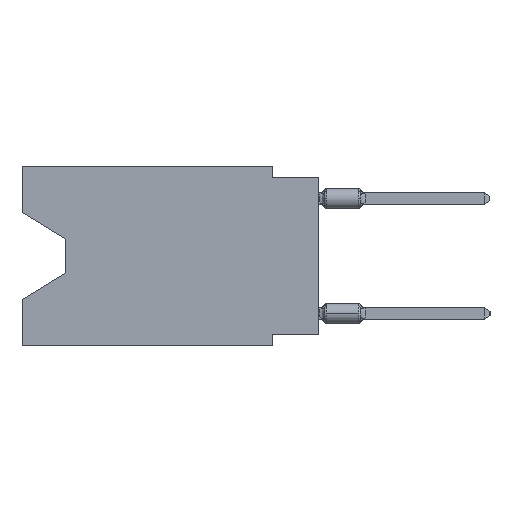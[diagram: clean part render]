
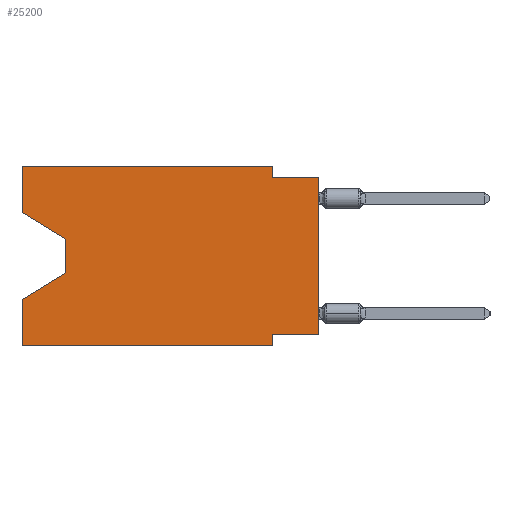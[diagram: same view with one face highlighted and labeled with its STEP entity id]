
A CAD part, left-side view. The second image highlights one B-rep face of the part: STEP entity #25200.
In plain terms, the highlighted planar face has unit normal (-1, 0, 0).
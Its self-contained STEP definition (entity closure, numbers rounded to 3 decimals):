
#260 = VECTOR ( 'NONE', #6667, 1000. ) ;
#454 = EDGE_CURVE ( 'NONE', #11448, #11130, #2234, .T. ) ;
#1502 = EDGE_CURVE ( 'NONE', #12271, #10239, #15780, .T. ) ;
#1909 = VECTOR ( 'NONE', #20679, 1000. ) ;
#2165 = ORIENTED_EDGE ( 'NONE', *, *, #1502, .T. ) ;
#2206 = ORIENTED_EDGE ( 'NONE', *, *, #2248, .F. ) ;
#2234 = LINE ( 'NONE', #36126, #32923 ) ;
#2248 = EDGE_CURVE ( 'NONE', #7473, #11448, #11424, .T. ) ;
#3458 = LINE ( 'NONE', #6251, #7971 ) ;
#4123 = ORIENTED_EDGE ( 'NONE', *, *, #14112, .F. ) ;
#4466 = CARTESIAN_POINT ( 'NONE',  ( 0., 13.97, -4.013 ) ) ;
#4873 = DIRECTION ( 'NONE',  ( 0., 0., -1. ) ) ;
#5042 = VECTOR ( 'NONE', #34159, 1000. ) ;
#5079 = VECTOR ( 'NONE', #7875, 1000. ) ;
#5109 = CARTESIAN_POINT ( 'NONE',  ( 0., 16.383, -2.546 ) ) ;
#5145 = EDGE_CURVE ( 'NONE', #11130, #29030, #25120, .T. ) ;
#5317 = CARTESIAN_POINT ( 'NONE',  ( 0., 13.97, -5.893 ) ) ;
#6251 = CARTESIAN_POINT ( 'NONE',  ( 0., 16.383, 0. ) ) ;
#6667 = DIRECTION ( 'NONE',  ( 0., -1., 0. ) ) ;
#6865 = LINE ( 'NONE', #12619, #1909 ) ;
#7071 = DIRECTION ( 'NONE',  ( 0., 0., -1. ) ) ;
#7473 = VERTEX_POINT ( 'NONE', #35876 ) ;
#7667 = CARTESIAN_POINT ( 'NONE',  ( 0., 16.383, -7.36 ) ) ;
#7672 = DIRECTION ( 'NONE',  ( 1., 0., 0. ) ) ;
#7689 = VERTEX_POINT ( 'NONE', #17421 ) ;
#7839 = DIRECTION ( 'NONE',  ( 0., 0., -1. ) ) ;
#7875 = DIRECTION ( 'NONE',  ( 0., 1., 0. ) ) ;
#7919 = CARTESIAN_POINT ( 'NONE',  ( 0., 2.54, -9.906 ) ) ;
#7971 = VECTOR ( 'NONE', #25437, 1000. ) ;
#8649 = LINE ( 'NONE', #5317, #36386 ) ;
#10239 = VERTEX_POINT ( 'NONE', #7919 ) ;
#10853 = LINE ( 'NONE', #14024, #5079 ) ;
#11130 = VERTEX_POINT ( 'NONE', #29367 ) ;
#11178 = ORIENTED_EDGE ( 'NONE', *, *, #29796, .T. ) ;
#11386 = EDGE_CURVE ( 'NONE', #7689, #33909, #8649, .T. ) ;
#11424 = LINE ( 'NONE', #22794, #5042 ) ;
#11448 = VERTEX_POINT ( 'NONE', #16852 ) ;
#12246 = ORIENTED_EDGE ( 'NONE', *, *, #11386, .T. ) ;
#12271 = VERTEX_POINT ( 'NONE', #22539 ) ;
#12602 = CARTESIAN_POINT ( 'NONE',  ( 0., 16.383, -9.906 ) ) ;
#12619 = CARTESIAN_POINT ( 'NONE',  ( 0., 13.97, -4.013 ) ) ;
#12708 = ORIENTED_EDGE ( 'NONE', *, *, #14794, .F. ) ;
#13194 = ORIENTED_EDGE ( 'NONE', *, *, #454, .F. ) ;
#13580 = VERTEX_POINT ( 'NONE', #18131 ) ;
#13663 = LINE ( 'NONE', #5109, #35019 ) ;
#13727 = LINE ( 'NONE', #27718, #34110 ) ;
#14024 = CARTESIAN_POINT ( 'NONE',  ( 0., 0., -9.271 ) ) ;
#14112 = EDGE_CURVE ( 'NONE', #12271, #33909, #13727, .T. ) ;
#14414 = LINE ( 'NONE', #17218, #34481 ) ;
#14794 = EDGE_CURVE ( 'NONE', #16448, #7473, #3458, .T. ) ;
#15780 = LINE ( 'NONE', #12602, #260 ) ;
#15794 = VERTEX_POINT ( 'NONE', #21589 ) ;
#16395 = ORIENTED_EDGE ( 'NONE', *, *, #5145, .F. ) ;
#16448 = VERTEX_POINT ( 'NONE', #34512 ) ;
#16852 = CARTESIAN_POINT ( 'NONE',  ( 0., 2.54, 0. ) ) ;
#17218 = CARTESIAN_POINT ( 'NONE',  ( 0., 0., 0. ) ) ;
#17421 = CARTESIAN_POINT ( 'NONE',  ( 0., 13.97, -5.893 ) ) ;
#17986 = EDGE_CURVE ( 'NONE', #13580, #15794, #10853, .T. ) ;
#18131 = CARTESIAN_POINT ( 'NONE',  ( 0., 0., -9.271 ) ) ;
#19537 = CARTESIAN_POINT ( 'NONE',  ( 0., 0., -0.635 ) ) ;
#19912 = EDGE_CURVE ( 'NONE', #15794, #10239, #22007, .T. ) ;
#20244 = VERTEX_POINT ( 'NONE', #4466 ) ;
#20679 = DIRECTION ( 'NONE',  ( 0., 0., -1. ) ) ;
#21148 = ORIENTED_EDGE ( 'NONE', *, *, #17986, .F. ) ;
#21589 = CARTESIAN_POINT ( 'NONE',  ( 0., 2.54, -9.271 ) ) ;
#21832 = PLANE ( 'NONE',  #27217 ) ;
#22007 = LINE ( 'NONE', #33358, #23028 ) ;
#22063 = ORIENTED_EDGE ( 'NONE', *, *, #19912, .F. ) ;
#22539 = CARTESIAN_POINT ( 'NONE',  ( 0., 16.383, -9.906 ) ) ;
#22794 = CARTESIAN_POINT ( 'NONE',  ( 0., 16.383, 0. ) ) ;
#23028 = VECTOR ( 'NONE', #7839, 1000. ) ;
#23331 = ORIENTED_EDGE ( 'NONE', *, *, #26347, .T. ) ;
#23971 = VECTOR ( 'NONE', #25312, 1000. ) ;
#25120 = LINE ( 'NONE', #19537, #23971 ) ;
#25200 = ADVANCED_FACE ( 'NONE', ( #33009 ), #21832, .F. ) ;
#25312 = DIRECTION ( 'NONE',  ( 0., -1., 0. ) ) ;
#25437 = DIRECTION ( 'NONE',  ( 0., 0., 1. ) ) ;
#25942 = EDGE_LOOP ( 'NONE', ( #23331, #30144, #12246, #4123, #2165, #22063, #21148, #11178, #16395, #13194, #2206, #12708 ) ) ;
#26347 = EDGE_CURVE ( 'NONE', #16448, #20244, #13663, .T. ) ;
#27217 = AXIS2_PLACEMENT_3D ( 'NONE', #33194, #7672, #4873 ) ;
#27718 = CARTESIAN_POINT ( 'NONE',  ( 0., 16.383, 0. ) ) ;
#27849 = DIRECTION ( 'NONE',  ( 0., 0.855, -0.519 ) ) ;
#29030 = VERTEX_POINT ( 'NONE', #30576 ) ;
#29367 = CARTESIAN_POINT ( 'NONE',  ( 0., 2.54, -0.635 ) ) ;
#29796 = EDGE_CURVE ( 'NONE', #13580, #29030, #14414, .T. ) ;
#30144 = ORIENTED_EDGE ( 'NONE', *, *, #35735, .T. ) ;
#30576 = CARTESIAN_POINT ( 'NONE',  ( 0., 0., -0.635 ) ) ;
#32923 = VECTOR ( 'NONE', #7071, 1000. ) ;
#33009 = FACE_OUTER_BOUND ( 'NONE', #25942, .T. ) ;
#33194 = CARTESIAN_POINT ( 'NONE',  ( 0., 16.383, 0. ) ) ;
#33358 = CARTESIAN_POINT ( 'NONE',  ( 0., 2.54, -9.906 ) ) ;
#33909 = VERTEX_POINT ( 'NONE', #7667 ) ;
#33957 = DIRECTION ( 'NONE',  ( 0., -0.855, -0.519 ) ) ;
#34032 = DIRECTION ( 'NONE',  ( 0., 0., 1. ) ) ;
#34110 = VECTOR ( 'NONE', #34032, 1000. ) ;
#34159 = DIRECTION ( 'NONE',  ( 0., -1., 0. ) ) ;
#34481 = VECTOR ( 'NONE', #36390, 1000. ) ;
#34512 = CARTESIAN_POINT ( 'NONE',  ( 0., 16.383, -2.546 ) ) ;
#35019 = VECTOR ( 'NONE', #33957, 1000. ) ;
#35735 = EDGE_CURVE ( 'NONE', #20244, #7689, #6865, .T. ) ;
#35876 = CARTESIAN_POINT ( 'NONE',  ( 0., 16.383, 0. ) ) ;
#36126 = CARTESIAN_POINT ( 'NONE',  ( 0., 2.54, 0. ) ) ;
#36386 = VECTOR ( 'NONE', #27849, 1000. ) ;
#36390 = DIRECTION ( 'NONE',  ( 0., 0., 1. ) ) ;
